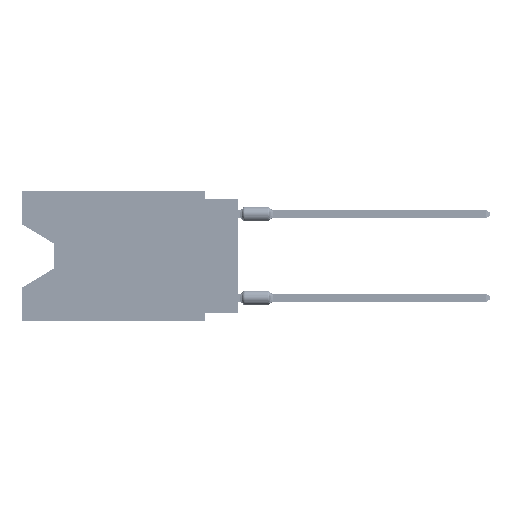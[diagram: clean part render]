
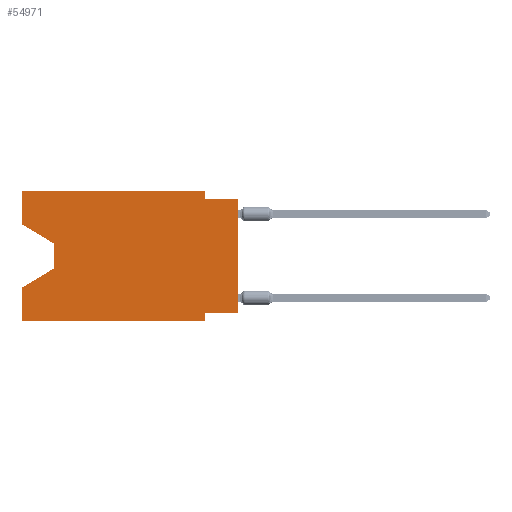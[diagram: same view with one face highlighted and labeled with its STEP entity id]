
A CAD part, left-side view. The second image highlights one B-rep face of the part: STEP entity #54971.
In plain terms, the highlighted planar face has unit normal (-1, 0, 0).
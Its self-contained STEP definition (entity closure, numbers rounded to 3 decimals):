
#2469 = LINE ( 'NONE', #8162, #33114 ) ;
#3193 = EDGE_CURVE ( 'NONE', #15309, #46435, #52687, .T. ) ;
#4925 = EDGE_CURVE ( 'NONE', #40007, #40494, #9441, .T. ) ;
#5375 = DIRECTION ( 'NONE',  ( 0., -1., 0. ) ) ;
#5940 = VECTOR ( 'NONE', #32910, 1000. ) ;
#6085 = CARTESIAN_POINT ( 'NONE',  ( 0., 0., -0.635 ) ) ;
#6120 = VECTOR ( 'NONE', #17096, 1000. ) ;
#7432 = LINE ( 'NONE', #39178, #58003 ) ;
#8162 = CARTESIAN_POINT ( 'NONE',  ( 0., 16.383, -9.906 ) ) ;
#9083 = CARTESIAN_POINT ( 'NONE',  ( 0., 16.383, 0. ) ) ;
#9441 = LINE ( 'NONE', #26169, #50682 ) ;
#11005 = VERTEX_POINT ( 'NONE', #54201 ) ;
#11974 = LINE ( 'NONE', #61848, #40785 ) ;
#13933 = ORIENTED_EDGE ( 'NONE', *, *, #19728, .F. ) ;
#14000 = VECTOR ( 'NONE', #55002, 1000. ) ;
#14417 = PLANE ( 'NONE',  #26234 ) ;
#15306 = ORIENTED_EDGE ( 'NONE', *, *, #51199, .F. ) ;
#15309 = VERTEX_POINT ( 'NONE', #20492 ) ;
#16732 = CARTESIAN_POINT ( 'NONE',  ( 0., 2.54, -9.906 ) ) ;
#16794 = CARTESIAN_POINT ( 'NONE',  ( 0., 0., -0.635 ) ) ;
#17096 = DIRECTION ( 'NONE',  ( 0., 0., -1. ) ) ;
#18976 = CARTESIAN_POINT ( 'NONE',  ( 0., 2.54, -9.271 ) ) ;
#19728 = EDGE_CURVE ( 'NONE', #35181, #34409, #64971, .T. ) ;
#20492 = CARTESIAN_POINT ( 'NONE',  ( 0., 0., -9.271 ) ) ;
#20540 = EDGE_CURVE ( 'NONE', #46435, #11005, #32776, .T. ) ;
#21444 = CARTESIAN_POINT ( 'NONE',  ( 0., 16.383, -9.906 ) ) ;
#22459 = LINE ( 'NONE', #44225, #47510 ) ;
#22925 = ORIENTED_EDGE ( 'NONE', *, *, #27286, .F. ) ;
#23558 = ORIENTED_EDGE ( 'NONE', *, *, #64214, .T. ) ;
#24411 = CARTESIAN_POINT ( 'NONE',  ( 0., 16.383, 0. ) ) ;
#24576 = VERTEX_POINT ( 'NONE', #16794 ) ;
#25122 = DIRECTION ( 'NONE',  ( 0., 0., 1. ) ) ;
#25259 = CARTESIAN_POINT ( 'NONE',  ( 0., 13.97, -5.893 ) ) ;
#25318 = LINE ( 'NONE', #63459, #35200 ) ;
#26024 = EDGE_LOOP ( 'NONE', ( #23558, #48383, #53976, #54093, #60424, #69958, #33709, #30038, #50426, #15306, #22925, #13933 ) ) ;
#26169 = CARTESIAN_POINT ( 'NONE',  ( 0., 13.97, -5.893 ) ) ;
#26234 = AXIS2_PLACEMENT_3D ( 'NONE', #9083, #30806, #52553 ) ;
#27286 = EDGE_CURVE ( 'NONE', #34409, #55449, #25318, .T. ) ;
#27563 = CARTESIAN_POINT ( 'NONE',  ( 0., 0., 0. ) ) ;
#28041 = CARTESIAN_POINT ( 'NONE',  ( 0., 16.383, 0. ) ) ;
#28954 = CARTESIAN_POINT ( 'NONE',  ( 0., 16.383, 0. ) ) ;
#30038 = ORIENTED_EDGE ( 'NONE', *, *, #44994, .T. ) ;
#30538 = VERTEX_POINT ( 'NONE', #60211 ) ;
#30806 = DIRECTION ( 'NONE',  ( 1., 0., 0. ) ) ;
#32776 = LINE ( 'NONE', #16732, #6120 ) ;
#32910 = DIRECTION ( 'NONE',  ( 0., 0., 1. ) ) ;
#33114 = VECTOR ( 'NONE', #52336, 1000. ) ;
#33709 = ORIENTED_EDGE ( 'NONE', *, *, #3193, .F. ) ;
#34409 = VERTEX_POINT ( 'NONE', #28041 ) ;
#35181 = VERTEX_POINT ( 'NONE', #43469 ) ;
#35200 = VECTOR ( 'NONE', #47419, 1000. ) ;
#35248 = CARTESIAN_POINT ( 'NONE',  ( 0., 0., -9.271 ) ) ;
#36182 = DIRECTION ( 'NONE',  ( 0., 0.855, -0.519 ) ) ;
#36402 = VERTEX_POINT ( 'NONE', #66365 ) ;
#36425 = LINE ( 'NONE', #6085, #70252 ) ;
#36845 = VECTOR ( 'NONE', #25122, 1000. ) ;
#39178 = CARTESIAN_POINT ( 'NONE',  ( 0., 13.97, -4.013 ) ) ;
#40007 = VERTEX_POINT ( 'NONE', #25259 ) ;
#40494 = VERTEX_POINT ( 'NONE', #67036 ) ;
#40785 = VECTOR ( 'NONE', #50116, 1000. ) ;
#41321 = EDGE_CURVE ( 'NONE', #43214, #40494, #68271, .T. ) ;
#43214 = VERTEX_POINT ( 'NONE', #21444 ) ;
#43469 = CARTESIAN_POINT ( 'NONE',  ( 0., 16.383, -2.546 ) ) ;
#44225 = CARTESIAN_POINT ( 'NONE',  ( 0., 2.54, 0. ) ) ;
#44994 = EDGE_CURVE ( 'NONE', #15309, #24576, #62013, .T. ) ;
#45939 = DIRECTION ( 'NONE',  ( 0., 1., 0. ) ) ;
#46435 = VERTEX_POINT ( 'NONE', #18976 ) ;
#47419 = DIRECTION ( 'NONE',  ( 0., -1., 0. ) ) ;
#47461 = CARTESIAN_POINT ( 'NONE',  ( 0., 2.54, 0. ) ) ;
#47510 = VECTOR ( 'NONE', #64885, 1000. ) ;
#48383 = ORIENTED_EDGE ( 'NONE', *, *, #66798, .T. ) ;
#49213 = VECTOR ( 'NONE', #45939, 1000. ) ;
#50116 = DIRECTION ( 'NONE',  ( 0., -0.855, -0.519 ) ) ;
#50426 = ORIENTED_EDGE ( 'NONE', *, *, #51144, .F. ) ;
#50682 = VECTOR ( 'NONE', #36182, 1000. ) ;
#51144 = EDGE_CURVE ( 'NONE', #30538, #24576, #36425, .T. ) ;
#51199 = EDGE_CURVE ( 'NONE', #55449, #30538, #22459, .T. ) ;
#52336 = DIRECTION ( 'NONE',  ( 0., -1., 0. ) ) ;
#52553 = DIRECTION ( 'NONE',  ( 0., 0., -1. ) ) ;
#52687 = LINE ( 'NONE', #35248, #49213 ) ;
#53976 = ORIENTED_EDGE ( 'NONE', *, *, #4925, .T. ) ;
#54093 = ORIENTED_EDGE ( 'NONE', *, *, #41321, .F. ) ;
#54201 = CARTESIAN_POINT ( 'NONE',  ( 0., 2.54, -9.906 ) ) ;
#54971 = ADVANCED_FACE ( 'NONE', ( #58929 ), #14417, .F. ) ;
#55002 = DIRECTION ( 'NONE',  ( 0., 0., 1. ) ) ;
#55449 = VERTEX_POINT ( 'NONE', #47461 ) ;
#58003 = VECTOR ( 'NONE', #60541, 1000. ) ;
#58929 = FACE_OUTER_BOUND ( 'NONE', #26024, .T. ) ;
#60211 = CARTESIAN_POINT ( 'NONE',  ( 0., 2.54, -0.635 ) ) ;
#60424 = ORIENTED_EDGE ( 'NONE', *, *, #68023, .T. ) ;
#60541 = DIRECTION ( 'NONE',  ( 0., 0., -1. ) ) ;
#61848 = CARTESIAN_POINT ( 'NONE',  ( 0., 16.383, -2.546 ) ) ;
#62013 = LINE ( 'NONE', #27563, #5940 ) ;
#63459 = CARTESIAN_POINT ( 'NONE',  ( 0., 16.383, 0. ) ) ;
#64214 = EDGE_CURVE ( 'NONE', #35181, #36402, #11974, .T. ) ;
#64885 = DIRECTION ( 'NONE',  ( 0., 0., -1. ) ) ;
#64971 = LINE ( 'NONE', #28954, #14000 ) ;
#66365 = CARTESIAN_POINT ( 'NONE',  ( 0., 13.97, -4.013 ) ) ;
#66798 = EDGE_CURVE ( 'NONE', #36402, #40007, #7432, .T. ) ;
#67036 = CARTESIAN_POINT ( 'NONE',  ( 0., 16.383, -7.36 ) ) ;
#68023 = EDGE_CURVE ( 'NONE', #43214, #11005, #2469, .T. ) ;
#68271 = LINE ( 'NONE', #24411, #36845 ) ;
#69958 = ORIENTED_EDGE ( 'NONE', *, *, #20540, .F. ) ;
#70252 = VECTOR ( 'NONE', #5375, 1000. ) ;
